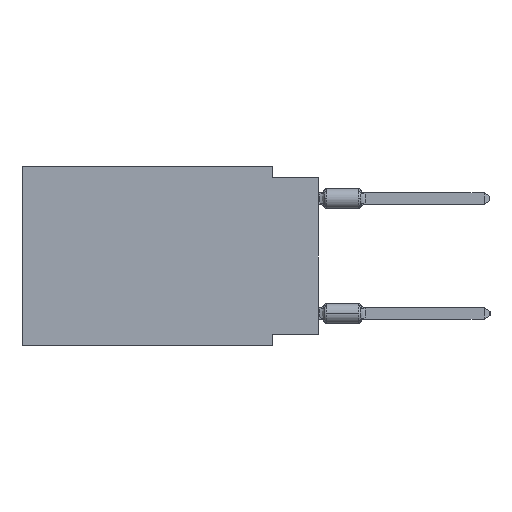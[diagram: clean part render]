
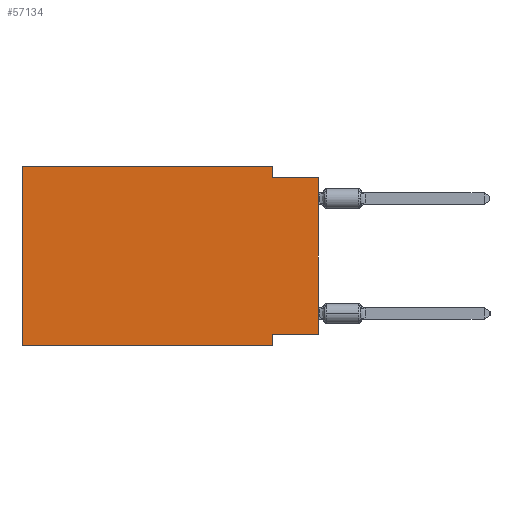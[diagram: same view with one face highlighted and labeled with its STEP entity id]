
A CAD part, left-side view. The second image highlights one B-rep face of the part: STEP entity #57134.
In plain terms, the highlighted planar face has unit normal (-1, 0, 0).
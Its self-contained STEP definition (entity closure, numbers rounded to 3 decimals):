
#60 = CARTESIAN_POINT ( 'NONE',  ( 0., 16.383, 0. ) ) ;
#174 = CARTESIAN_POINT ( 'NONE',  ( 0., 0., 0. ) ) ;
#3304 = VECTOR ( 'NONE', #22052, 1000. ) ;
#3344 = DIRECTION ( 'NONE',  ( 0., 0., -1. ) ) ;
#3935 = VECTOR ( 'NONE', #52844, 1000. ) ;
#4299 = CARTESIAN_POINT ( 'NONE',  ( 0., 16.383, 0. ) ) ;
#4953 = LINE ( 'NONE', #174, #3304 ) ;
#7097 = EDGE_CURVE ( 'NONE', #31954, #40151, #43739, .T. ) ;
#7739 = CARTESIAN_POINT ( 'NONE',  ( 0., 0., -9.271 ) ) ;
#8306 = EDGE_CURVE ( 'NONE', #31954, #34076, #52225, .T. ) ;
#9562 = VERTEX_POINT ( 'NONE', #30659 ) ;
#11095 = VERTEX_POINT ( 'NONE', #58338 ) ;
#11149 = CARTESIAN_POINT ( 'NONE',  ( 0., 0., -9.271 ) ) ;
#12567 = ORIENTED_EDGE ( 'NONE', *, *, #42114, .F. ) ;
#13046 = CARTESIAN_POINT ( 'NONE',  ( 0., 2.54, -9.271 ) ) ;
#15358 = VECTOR ( 'NONE', #38439, 1000. ) ;
#16185 = DIRECTION ( 'NONE',  ( 0., -1., 0. ) ) ;
#16627 = ORIENTED_EDGE ( 'NONE', *, *, #7097, .T. ) ;
#17772 = PLANE ( 'NONE',  #55975 ) ;
#20797 = CARTESIAN_POINT ( 'NONE',  ( 0., 0., -0.635 ) ) ;
#22052 = DIRECTION ( 'NONE',  ( 0., 0., 1. ) ) ;
#23678 = EDGE_CURVE ( 'NONE', #37460, #9562, #4953, .T. ) ;
#24735 = ORIENTED_EDGE ( 'NONE', *, *, #23678, .T. ) ;
#25307 = VECTOR ( 'NONE', #3344, 1000. ) ;
#27002 = LINE ( 'NONE', #35702, #25307 ) ;
#27062 = DIRECTION ( 'NONE',  ( 1., 0., 0. ) ) ;
#27127 = CARTESIAN_POINT ( 'NONE',  ( 0., 2.54, -9.906 ) ) ;
#28768 = ORIENTED_EDGE ( 'NONE', *, *, #29634, .F. ) ;
#29634 = EDGE_CURVE ( 'NONE', #48097, #40151, #48121, .T. ) ;
#30169 = DIRECTION ( 'NONE',  ( 0., 0., -1. ) ) ;
#30659 = CARTESIAN_POINT ( 'NONE',  ( 0., 0., -0.635 ) ) ;
#31565 = DIRECTION ( 'NONE',  ( 0., 0., -1. ) ) ;
#31954 = VERTEX_POINT ( 'NONE', #32434 ) ;
#32434 = CARTESIAN_POINT ( 'NONE',  ( 0., 16.383, -9.906 ) ) ;
#32534 = ORIENTED_EDGE ( 'NONE', *, *, #43161, .F. ) ;
#33678 = CARTESIAN_POINT ( 'NONE',  ( 0., 16.383, 0. ) ) ;
#34076 = VERTEX_POINT ( 'NONE', #60 ) ;
#34672 = CARTESIAN_POINT ( 'NONE',  ( 0., 2.54, -9.906 ) ) ;
#35576 = ORIENTED_EDGE ( 'NONE', *, *, #8306, .F. ) ;
#35702 = CARTESIAN_POINT ( 'NONE',  ( 0., 2.54, 0. ) ) ;
#36059 = FACE_OUTER_BOUND ( 'NONE', #58891, .T. ) ;
#37460 = VERTEX_POINT ( 'NONE', #7739 ) ;
#37767 = VERTEX_POINT ( 'NONE', #44507 ) ;
#37962 = CARTESIAN_POINT ( 'NONE',  ( 0., 16.383, 0. ) ) ;
#38439 = DIRECTION ( 'NONE',  ( 0., 0., 1. ) ) ;
#38753 = ORIENTED_EDGE ( 'NONE', *, *, #52188, .F. ) ;
#39899 = VECTOR ( 'NONE', #30169, 1000. ) ;
#40151 = VERTEX_POINT ( 'NONE', #27127 ) ;
#41854 = DIRECTION ( 'NONE',  ( 0., -1., 0. ) ) ;
#42114 = EDGE_CURVE ( 'NONE', #34076, #11095, #42741, .T. ) ;
#42368 = VECTOR ( 'NONE', #41854, 1000. ) ;
#42741 = LINE ( 'NONE', #37962, #42368 ) ;
#43161 = EDGE_CURVE ( 'NONE', #37460, #48097, #43189, .T. ) ;
#43189 = LINE ( 'NONE', #11149, #45266 ) ;
#43739 = LINE ( 'NONE', #48224, #58307 ) ;
#44485 = EDGE_CURVE ( 'NONE', #11095, #37767, #27002, .T. ) ;
#44507 = CARTESIAN_POINT ( 'NONE',  ( 0., 2.54, -0.635 ) ) ;
#45266 = VECTOR ( 'NONE', #57557, 1000. ) ;
#48097 = VERTEX_POINT ( 'NONE', #13046 ) ;
#48121 = LINE ( 'NONE', #34672, #39899 ) ;
#48224 = CARTESIAN_POINT ( 'NONE',  ( 0., 16.383, -9.906 ) ) ;
#48932 = LINE ( 'NONE', #20797, #3935 ) ;
#52188 = EDGE_CURVE ( 'NONE', #37767, #9562, #48932, .T. ) ;
#52225 = LINE ( 'NONE', #33678, #15358 ) ;
#52844 = DIRECTION ( 'NONE',  ( 0., -1., 0. ) ) ;
#55250 = ORIENTED_EDGE ( 'NONE', *, *, #44485, .F. ) ;
#55975 = AXIS2_PLACEMENT_3D ( 'NONE', #4299, #27062, #31565 ) ;
#57134 = ADVANCED_FACE ( 'NONE', ( #36059 ), #17772, .F. ) ;
#57557 = DIRECTION ( 'NONE',  ( 0., 1., 0. ) ) ;
#58307 = VECTOR ( 'NONE', #16185, 1000. ) ;
#58338 = CARTESIAN_POINT ( 'NONE',  ( 0., 2.54, 0. ) ) ;
#58891 = EDGE_LOOP ( 'NONE', ( #24735, #38753, #55250, #12567, #35576, #16627, #28768, #32534 ) ) ;
